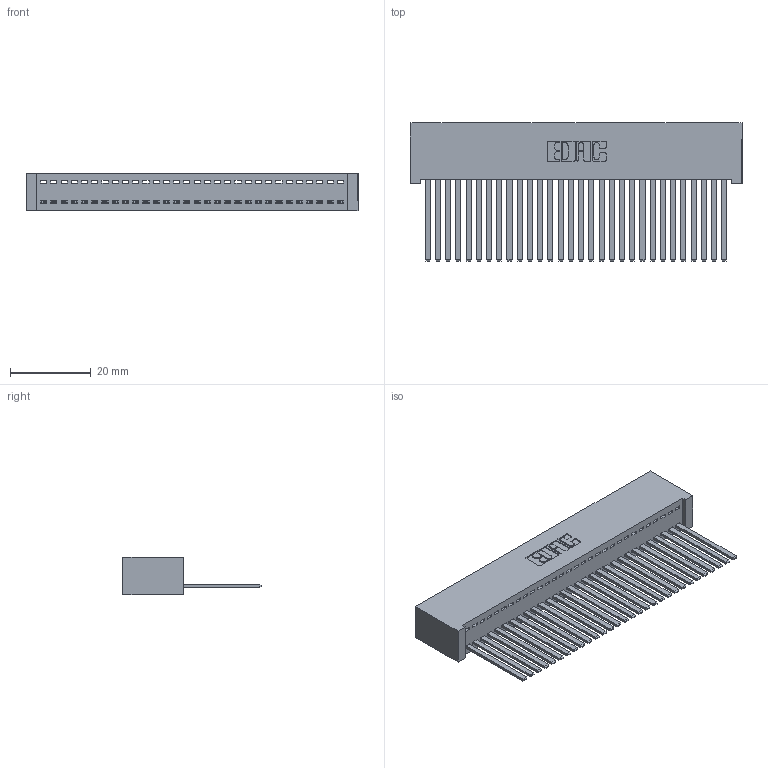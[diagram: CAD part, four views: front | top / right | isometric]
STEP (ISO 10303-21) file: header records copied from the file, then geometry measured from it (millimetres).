
FILE_DESCRIPTION (( 'STEP AP203' ), '1' );
FILE_NAME ('392-030-544-101.STEP', '2018-08-15T22:39:31', ( '' ), ( '' ), 'SwSTEP 2.0', 'SolidWorks 2016', '' );
FILE_SCHEMA (( 'CONFIG_CONTROL_DESIGN' ));
Length unit declared in the file: inch
Products named in the file (3): 342 Part_Lugless; 345-292-001_345-293-144; 392-030-544-101
Assembly tree (31 placements, depth 2):
  392-030-544-101
    342 Part_Lugless
    345-292-001_345-293-144  x30
Bounding box: 82.45 x 34.3 x 9.4 mm (x, y, z)
Volume: 7941.3 mm3; surface area: 12749.5 mm2
Topology: 31 solids, 31 shells, 1662 faces, 5015 edges, 3302 vertices
Faces by surface type: plane 1202, cylinder 460
Entity records: 19299 total; most frequent: CARTESIAN_POINT 3336, ORIENTED_EDGE 3302, DIRECTION 2827, EDGE_CURVE 1651, LINE 1535, VECTOR 1535, VERTEX_POINT 1098, AXIS2_PLACEMENT_3D 646
